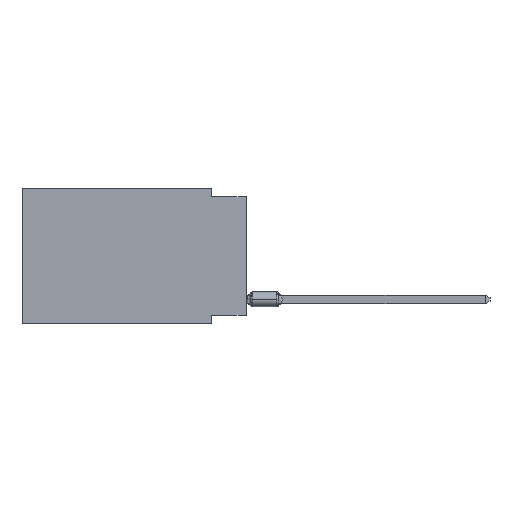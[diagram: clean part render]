
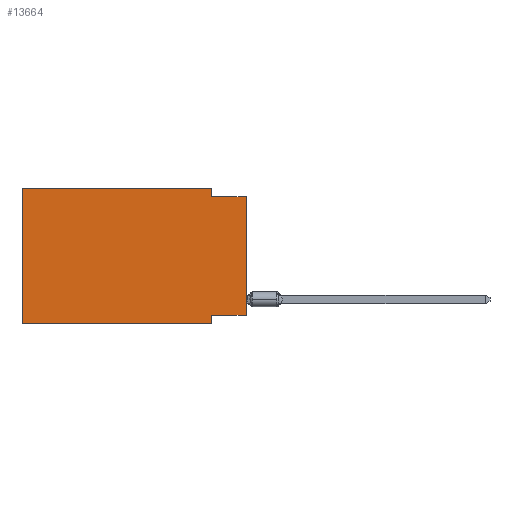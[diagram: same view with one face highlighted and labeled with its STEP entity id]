
A CAD part, left-side view. The second image highlights one B-rep face of the part: STEP entity #13664.
In plain terms, the highlighted planar face has unit normal (-1, 0, 0).
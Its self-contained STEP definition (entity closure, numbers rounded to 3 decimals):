
#161 = ORIENTED_EDGE ( 'NONE', *, *, #3997, .T. ) ;
#274 = ORIENTED_EDGE ( 'NONE', *, *, #14788, .F. ) ;
#351 = DIRECTION ( 'NONE',  ( 0., 0., 1. ) ) ;
#507 = ORIENTED_EDGE ( 'NONE', *, *, #10486, .F. ) ;
#1010 = VERTEX_POINT ( 'NONE', #5199 ) ;
#1125 = CARTESIAN_POINT ( 'NONE',  ( 0., 16.383, -9.906 ) ) ;
#1159 = VERTEX_POINT ( 'NONE', #12113 ) ;
#1185 = EDGE_CURVE ( 'NONE', #13826, #13321, #13689, .T. ) ;
#1408 = CARTESIAN_POINT ( 'NONE',  ( 0., 0., -0.635 ) ) ;
#1432 = VERTEX_POINT ( 'NONE', #1408 ) ;
#1722 = VERTEX_POINT ( 'NONE', #4396 ) ;
#1787 = VECTOR ( 'NONE', #15086, 1000. ) ;
#2028 = VERTEX_POINT ( 'NONE', #12311 ) ;
#2112 = CARTESIAN_POINT ( 'NONE',  ( 0., 16.383, 0. ) ) ;
#2306 = VECTOR ( 'NONE', #4609, 1000. ) ;
#2461 = LINE ( 'NONE', #13391, #4225 ) ;
#2546 = LINE ( 'NONE', #7117, #10560 ) ;
#2684 = AXIS2_PLACEMENT_3D ( 'NONE', #9725, #11922, #11062 ) ;
#2958 = VECTOR ( 'NONE', #4160, 1000. ) ;
#3211 = PLANE ( 'NONE',  #2684 ) ;
#3862 = VECTOR ( 'NONE', #351, 1000. ) ;
#3997 = EDGE_CURVE ( 'NONE', #1722, #1432, #8920, .T. ) ;
#4160 = DIRECTION ( 'NONE',  ( 0., -1., 0. ) ) ;
#4225 = VECTOR ( 'NONE', #12047, 1000. ) ;
#4273 = ORIENTED_EDGE ( 'NONE', *, *, #6486, .T. ) ;
#4396 = CARTESIAN_POINT ( 'NONE',  ( 0., 0., -9.271 ) ) ;
#4523 = EDGE_CURVE ( 'NONE', #1159, #2028, #8628, .T. ) ;
#4609 = DIRECTION ( 'NONE',  ( 0., -1., 0. ) ) ;
#5101 = CARTESIAN_POINT ( 'NONE',  ( 0., 2.54, -9.271 ) ) ;
#5199 = CARTESIAN_POINT ( 'NONE',  ( 0., 2.54, -0.635 ) ) ;
#5896 = LINE ( 'NONE', #2112, #14323 ) ;
#6486 = EDGE_CURVE ( 'NONE', #11917, #13321, #11669, .T. ) ;
#7117 = CARTESIAN_POINT ( 'NONE',  ( 0., 0., -9.271 ) ) ;
#7737 = CARTESIAN_POINT ( 'NONE',  ( 0., 0., 0. ) ) ;
#8090 = DIRECTION ( 'NONE',  ( 0., 0., 1. ) ) ;
#8315 = VECTOR ( 'NONE', #9481, 1000. ) ;
#8425 = CARTESIAN_POINT ( 'NONE',  ( 0., 2.54, -9.906 ) ) ;
#8628 = LINE ( 'NONE', #13310, #8315 ) ;
#8920 = LINE ( 'NONE', #7737, #3862 ) ;
#9481 = DIRECTION ( 'NONE',  ( 0., -1., 0. ) ) ;
#9725 = CARTESIAN_POINT ( 'NONE',  ( 0., 16.383, 0. ) ) ;
#9960 = CARTESIAN_POINT ( 'NONE',  ( 0., 0., -0.635 ) ) ;
#10254 = ORIENTED_EDGE ( 'NONE', *, *, #15173, .F. ) ;
#10317 = ORIENTED_EDGE ( 'NONE', *, *, #4523, .F. ) ;
#10486 = EDGE_CURVE ( 'NONE', #11917, #1159, #5896, .T. ) ;
#10560 = VECTOR ( 'NONE', #11818, 1000. ) ;
#11062 = DIRECTION ( 'NONE',  ( 0., 0., -1. ) ) ;
#11264 = CARTESIAN_POINT ( 'NONE',  ( 0., 2.54, -9.906 ) ) ;
#11539 = FACE_OUTER_BOUND ( 'NONE', #14899, .T. ) ;
#11669 = LINE ( 'NONE', #1125, #2306 ) ;
#11701 = ORIENTED_EDGE ( 'NONE', *, *, #12938, .F. ) ;
#11818 = DIRECTION ( 'NONE',  ( 0., 1., 0. ) ) ;
#11917 = VERTEX_POINT ( 'NONE', #14532 ) ;
#11922 = DIRECTION ( 'NONE',  ( 1., 0., 0. ) ) ;
#12047 = DIRECTION ( 'NONE',  ( 0., 0., -1. ) ) ;
#12113 = CARTESIAN_POINT ( 'NONE',  ( 0., 16.383, 0. ) ) ;
#12311 = CARTESIAN_POINT ( 'NONE',  ( 0., 2.54, 0. ) ) ;
#12938 = EDGE_CURVE ( 'NONE', #1722, #13826, #2546, .T. ) ;
#13310 = CARTESIAN_POINT ( 'NONE',  ( 0., 16.383, 0. ) ) ;
#13321 = VERTEX_POINT ( 'NONE', #8425 ) ;
#13391 = CARTESIAN_POINT ( 'NONE',  ( 0., 2.54, 0. ) ) ;
#13664 = ADVANCED_FACE ( 'NONE', ( #11539 ), #3211, .F. ) ;
#13689 = LINE ( 'NONE', #11264, #1787 ) ;
#13826 = VERTEX_POINT ( 'NONE', #5101 ) ;
#14323 = VECTOR ( 'NONE', #8090, 1000. ) ;
#14532 = CARTESIAN_POINT ( 'NONE',  ( 0., 16.383, -9.906 ) ) ;
#14712 = ORIENTED_EDGE ( 'NONE', *, *, #1185, .F. ) ;
#14788 = EDGE_CURVE ( 'NONE', #1010, #1432, #14907, .T. ) ;
#14899 = EDGE_LOOP ( 'NONE', ( #161, #274, #10254, #10317, #507, #4273, #14712, #11701 ) ) ;
#14907 = LINE ( 'NONE', #9960, #2958 ) ;
#15086 = DIRECTION ( 'NONE',  ( 0., 0., -1. ) ) ;
#15173 = EDGE_CURVE ( 'NONE', #2028, #1010, #2461, .T. ) ;
